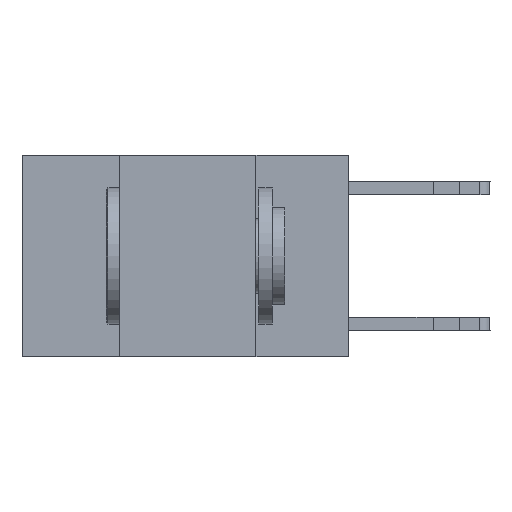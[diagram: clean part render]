
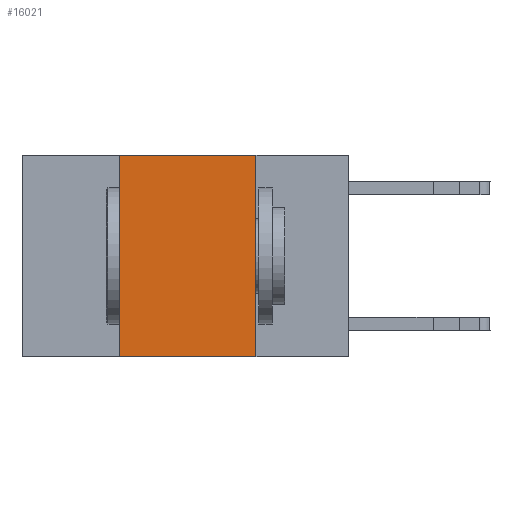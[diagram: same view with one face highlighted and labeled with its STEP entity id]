
A CAD part, left-side view. The second image highlights one B-rep face of the part: STEP entity #16021.
In plain terms, the highlighted planar face has unit normal (-1, 0, 0).
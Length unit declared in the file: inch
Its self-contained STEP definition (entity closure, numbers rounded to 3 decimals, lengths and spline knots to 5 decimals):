
#1149 = CARTESIAN_POINT ( 'NONE',  ( 0., 0.6, -0.37 ) ) ;
#1266 = DIRECTION ( 'NONE',  ( 0., -1., 0. ) ) ;
#1320 = DIRECTION ( 'NONE',  ( 0., 0., -1. ) ) ;
#1346 = CARTESIAN_POINT ( 'NONE',  ( 0., 0.42, 0. ) ) ;
#1867 = VECTOR ( 'NONE', #20680, 39.37008 ) ;
#2659 = FACE_OUTER_BOUND ( 'NONE', #16787, .T. ) ;
#2774 = DIRECTION ( 'NONE',  ( 1., 0., 0. ) ) ;
#4566 = VERTEX_POINT ( 'NONE', #10112 ) ;
#5034 = ORIENTED_EDGE ( 'NONE', *, *, #5076, .T. ) ;
#5076 = EDGE_CURVE ( 'NONE', #10515, #7749, #5130, .T. ) ;
#5130 = LINE ( 'NONE', #1149, #9240 ) ;
#6538 = ORIENTED_EDGE ( 'NONE', *, *, #12615, .F. ) ;
#7514 = DIRECTION ( 'NONE',  ( 0., -1., 0. ) ) ;
#7749 = VERTEX_POINT ( 'NONE', #9776 ) ;
#8159 = VECTOR ( 'NONE', #7514, 39.37008 ) ;
#9240 = VECTOR ( 'NONE', #1266, 39.37008 ) ;
#9513 = EDGE_CURVE ( 'NONE', #14964, #7749, #14328, .T. ) ;
#9729 = ORIENTED_EDGE ( 'NONE', *, *, #9513, .F. ) ;
#9776 = CARTESIAN_POINT ( 'NONE',  ( 0., 0.17, -0.37 ) ) ;
#10112 = CARTESIAN_POINT ( 'NONE',  ( 0., 0.42, 0. ) ) ;
#10191 = PLANE ( 'NONE',  #20964 ) ;
#10302 = DIRECTION ( 'NONE',  ( 0., 0., -1. ) ) ;
#10515 = VERTEX_POINT ( 'NONE', #13407 ) ;
#10881 = CARTESIAN_POINT ( 'NONE',  ( 0., 0.6, 0. ) ) ;
#12615 = EDGE_CURVE ( 'NONE', #4566, #14964, #16786, .T. ) ;
#13407 = CARTESIAN_POINT ( 'NONE',  ( 0., 0.42, -0.37 ) ) ;
#13732 = VECTOR ( 'NONE', #1320, 39.37008 ) ;
#14328 = LINE ( 'NONE', #20288, #13732 ) ;
#14964 = VERTEX_POINT ( 'NONE', #15329 ) ;
#15329 = CARTESIAN_POINT ( 'NONE',  ( 0., 0.17, 0. ) ) ;
#16021 = ADVANCED_FACE ( 'NONE', ( #2659 ), #10191, .F. ) ;
#16786 = LINE ( 'NONE', #10881, #8159 ) ;
#16787 = EDGE_LOOP ( 'NONE', ( #9729, #6538, #19062, #5034 ) ) ;
#17732 = CARTESIAN_POINT ( 'NONE',  ( 0., 0.6, 0. ) ) ;
#18195 = LINE ( 'NONE', #1346, #1867 ) ;
#19062 = ORIENTED_EDGE ( 'NONE', *, *, #21485, .F. ) ;
#20288 = CARTESIAN_POINT ( 'NONE',  ( 0., 0.17, 0. ) ) ;
#20680 = DIRECTION ( 'NONE',  ( 0., 0., 1. ) ) ;
#20964 = AXIS2_PLACEMENT_3D ( 'NONE', #17732, #2774, #10302 ) ;
#21485 = EDGE_CURVE ( 'NONE', #10515, #4566, #18195, .T. ) ;
